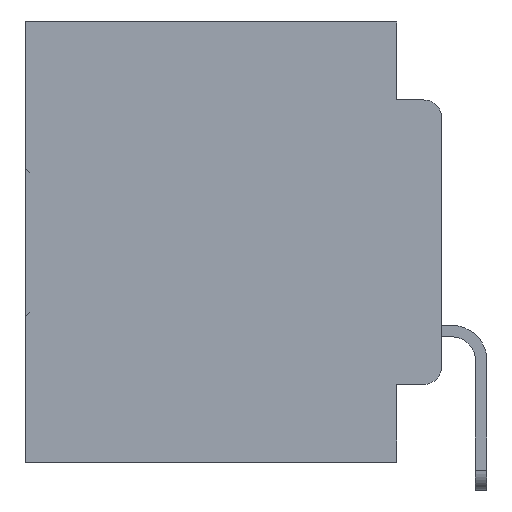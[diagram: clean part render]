
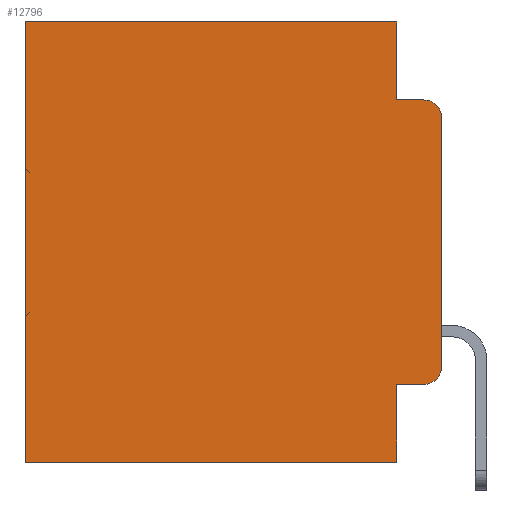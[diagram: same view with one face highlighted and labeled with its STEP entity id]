
A CAD part, left-side view. The second image highlights one B-rep face of the part: STEP entity #12796.
In plain terms, the highlighted planar face has unit normal (-1, 0, 0).
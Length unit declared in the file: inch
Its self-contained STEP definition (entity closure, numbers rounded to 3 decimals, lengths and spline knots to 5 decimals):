
#582 = LINE ( 'NONE', #1683, #13932 ) ;
#1251 = CARTESIAN_POINT ( 'NONE',  ( 0.298, 0.02, -0.4115 ) ) ;
#1279 = CARTESIAN_POINT ( 'NONE',  ( 0.298, 0., -0.1085 ) ) ;
#1486 = CARTESIAN_POINT ( 'NONE',  ( 0.298, 0., 0. ) ) ;
#1683 = CARTESIAN_POINT ( 'NONE',  ( 0.298, 0.051, -0.0885 ) ) ;
#1758 = CARTESIAN_POINT ( 'NONE',  ( 0.298, 0.02, -0.3915 ) ) ;
#1825 = CARTESIAN_POINT ( 'NONE',  ( 0.298, 0., 0. ) ) ;
#3897 = AXIS2_PLACEMENT_3D ( 'NONE', #1758, #21001, #4657 ) ;
#4591 = DIRECTION ( 'NONE',  ( 0., -1., 0. ) ) ;
#4657 = DIRECTION ( 'NONE',  ( 0., 0., -1. ) ) ;
#4731 = DIRECTION ( 'NONE',  ( 0., 0., -1. ) ) ;
#5687 = DIRECTION ( 'NONE',  ( 0., -1., 0. ) ) ;
#6429 = VECTOR ( 'NONE', #19030, 39.37008 ) ;
#7061 = VECTOR ( 'NONE', #28371, 39.37008 ) ;
#7644 = LINE ( 'NONE', #9815, #21095 ) ;
#8191 = ORIENTED_EDGE ( 'NONE', *, *, #12594, .T. ) ;
#8816 = EDGE_CURVE ( 'NONE', #22542, #9817, #19239, .T. ) ;
#9128 = LINE ( 'NONE', #24587, #17186 ) ;
#9171 = LINE ( 'NONE', #1486, #6429 ) ;
#9312 = CARTESIAN_POINT ( 'NONE',  ( 0.298, 0., -0.3915 ) ) ;
#9815 = CARTESIAN_POINT ( 'NONE',  ( 0.298, 0.473, 0. ) ) ;
#9817 = VERTEX_POINT ( 'NONE', #9312 ) ;
#10176 = VERTEX_POINT ( 'NONE', #26794 ) ;
#10348 = ORIENTED_EDGE ( 'NONE', *, *, #21352, .F. ) ;
#10585 = CARTESIAN_POINT ( 'NONE',  ( 0.298, 0.051, -0.4115 ) ) ;
#10934 = VERTEX_POINT ( 'NONE', #26018 ) ;
#12594 = EDGE_CURVE ( 'NONE', #17167, #22542, #9128, .T. ) ;
#12796 = ADVANCED_FACE ( 'NONE', ( #21197 ), #27624, .F. ) ;
#13242 = VERTEX_POINT ( 'NONE', #1279 ) ;
#13887 = CARTESIAN_POINT ( 'NONE',  ( 0.298, 0., -0.5 ) ) ;
#13932 = VECTOR ( 'NONE', #4591, 39.37008 ) ;
#14426 = EDGE_CURVE ( 'NONE', #17167, #27223, #26023, .T. ) ;
#14773 = ORIENTED_EDGE ( 'NONE', *, *, #8816, .T. ) ;
#14948 = DIRECTION ( 'NONE',  ( 0., 0., -1. ) ) ;
#15573 = ORIENTED_EDGE ( 'NONE', *, *, #14426, .F. ) ;
#15747 = DIRECTION ( 'NONE',  ( -1., 0., 0. ) ) ;
#16544 = DIRECTION ( 'NONE',  ( 0., 1., 0. ) ) ;
#17167 = VERTEX_POINT ( 'NONE', #10585 ) ;
#17186 = VECTOR ( 'NONE', #5687, 39.37008 ) ;
#17923 = EDGE_CURVE ( 'NONE', #29900, #10934, #7644, .T. ) ;
#18422 = LINE ( 'NONE', #13887, #31001 ) ;
#19030 = DIRECTION ( 'NONE',  ( 0., 1., 0. ) ) ;
#19239 = CIRCLE ( 'NONE', #3897, 0.02 ) ;
#19606 = EDGE_CURVE ( 'NONE', #28829, #10176, #21391, .T. ) ;
#20207 = ORIENTED_EDGE ( 'NONE', *, *, #32745, .T. ) ;
#20496 = LINE ( 'NONE', #1825, #32155 ) ;
#20738 = AXIS2_PLACEMENT_3D ( 'NONE', #22657, #30164, #14948 ) ;
#21001 = DIRECTION ( 'NONE',  ( -1., 0., 0. ) ) ;
#21095 = VECTOR ( 'NONE', #23048, 39.37008 ) ;
#21170 = ORIENTED_EDGE ( 'NONE', *, *, #33380, .F. ) ;
#21197 = FACE_OUTER_BOUND ( 'NONE', #29973, .T. ) ;
#21352 = EDGE_CURVE ( 'NONE', #10176, #29183, #582, .T. ) ;
#21391 = LINE ( 'NONE', #25947, #7061 ) ;
#21786 = CARTESIAN_POINT ( 'NONE',  ( 0.298, 0.02, -0.0885 ) ) ;
#22513 = DIRECTION ( 'NONE',  ( 0., 0., -1. ) ) ;
#22542 = VERTEX_POINT ( 'NONE', #1251 ) ;
#22657 = CARTESIAN_POINT ( 'NONE',  ( 0.298, 0., 0. ) ) ;
#23048 = DIRECTION ( 'NONE',  ( 0., 0., -1. ) ) ;
#24587 = CARTESIAN_POINT ( 'NONE',  ( 0.298, 0.051, -0.4115 ) ) ;
#25947 = CARTESIAN_POINT ( 'NONE',  ( 0.298, 0.051, 0. ) ) ;
#26018 = CARTESIAN_POINT ( 'NONE',  ( 0.298, 0.473, -0.5 ) ) ;
#26023 = LINE ( 'NONE', #27505, #31634 ) ;
#26519 = ORIENTED_EDGE ( 'NONE', *, *, #28163, .T. ) ;
#26794 = CARTESIAN_POINT ( 'NONE',  ( 0.298, 0.051, -0.0885 ) ) ;
#27006 = CARTESIAN_POINT ( 'NONE',  ( 0.298, 0.051, -0.5 ) ) ;
#27223 = VERTEX_POINT ( 'NONE', #27006 ) ;
#27505 = CARTESIAN_POINT ( 'NONE',  ( 0.298, 0.051, 0. ) ) ;
#27624 = PLANE ( 'NONE',  #20738 ) ;
#27999 = CARTESIAN_POINT ( 'NONE',  ( 0.298, 0.051, 0. ) ) ;
#28163 = EDGE_CURVE ( 'NONE', #13242, #29183, #30841, .T. ) ;
#28371 = DIRECTION ( 'NONE',  ( 0., 0., -1. ) ) ;
#28498 = ORIENTED_EDGE ( 'NONE', *, *, #19606, .F. ) ;
#28829 = VERTEX_POINT ( 'NONE', #27999 ) ;
#28997 = ORIENTED_EDGE ( 'NONE', *, *, #17923, .T. ) ;
#29183 = VERTEX_POINT ( 'NONE', #21786 ) ;
#29900 = VERTEX_POINT ( 'NONE', #32163 ) ;
#29973 = EDGE_LOOP ( 'NONE', ( #32462, #26519, #10348, #28498, #20207, #28997, #21170, #15573, #8191, #14773 ) ) ;
#30164 = DIRECTION ( 'NONE',  ( 1., 0., 0. ) ) ;
#30841 = CIRCLE ( 'NONE', #31254, 0.02 ) ;
#30899 = CARTESIAN_POINT ( 'NONE',  ( 0.298, 0.02, -0.1085 ) ) ;
#31001 = VECTOR ( 'NONE', #16544, 39.37008 ) ;
#31254 = AXIS2_PLACEMENT_3D ( 'NONE', #30899, #15747, #33261 ) ;
#31367 = EDGE_CURVE ( 'NONE', #13242, #9817, #20496, .T. ) ;
#31634 = VECTOR ( 'NONE', #22513, 39.37008 ) ;
#32155 = VECTOR ( 'NONE', #4731, 39.37008 ) ;
#32163 = CARTESIAN_POINT ( 'NONE',  ( 0.298, 0.473, 0. ) ) ;
#32462 = ORIENTED_EDGE ( 'NONE', *, *, #31367, .F. ) ;
#32745 = EDGE_CURVE ( 'NONE', #28829, #29900, #9171, .T. ) ;
#33261 = DIRECTION ( 'NONE',  ( 0., 0., -1. ) ) ;
#33380 = EDGE_CURVE ( 'NONE', #27223, #10934, #18422, .T. ) ;
